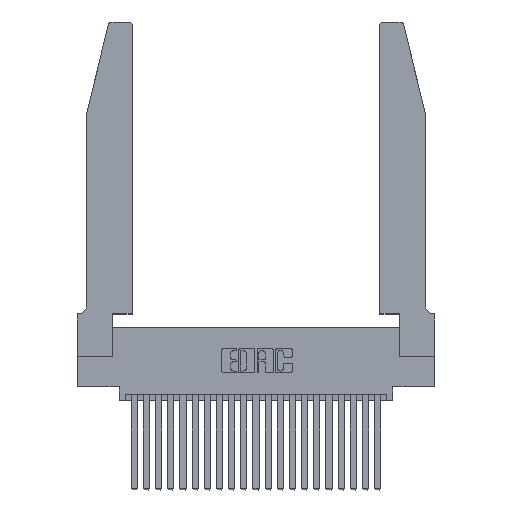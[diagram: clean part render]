
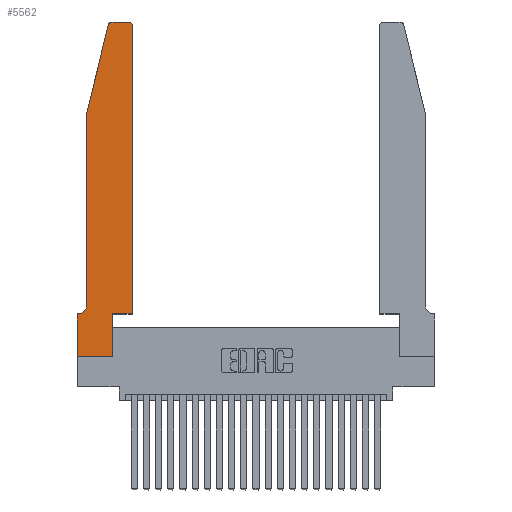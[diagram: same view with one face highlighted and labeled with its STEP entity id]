
A CAD part, top view. The second image highlights one B-rep face of the part: STEP entity #5562.
In plain terms, the highlighted planar face has unit normal (0, 0, 1).
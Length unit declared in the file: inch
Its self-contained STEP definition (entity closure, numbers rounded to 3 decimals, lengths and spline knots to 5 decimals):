
#149 = VECTOR ( 'NONE', #1515, 39.37008 ) ;
#479 = DIRECTION ( 'NONE',  ( 0., 0., 1. ) ) ;
#844 = EDGE_CURVE ( 'NONE', #2425, #8288, #3232, .T. ) ;
#851 = ORIENTED_EDGE ( 'NONE', *, *, #21443, .T. ) ;
#1072 = AXIS2_PLACEMENT_3D ( 'NONE', #11832, #479, #13638 ) ;
#1257 = EDGE_CURVE ( 'NONE', #16092, #20178, #22790, .T. ) ;
#1515 = DIRECTION ( 'NONE',  ( 0., 1., 0. ) ) ;
#1589 = EDGE_CURVE ( 'NONE', #8951, #5964, #16512, .T. ) ;
#1656 = VECTOR ( 'NONE', #19403, 39.37008 ) ;
#2425 = VERTEX_POINT ( 'NONE', #13610 ) ;
#2633 = CARTESIAN_POINT ( 'NONE',  ( 0.4205, 2.72, 0.37 ) ) ;
#2697 = ORIENTED_EDGE ( 'NONE', *, *, #7493, .T. ) ;
#2860 = DIRECTION ( 'NONE',  ( 0., 0., 1. ) ) ;
#3204 = AXIS2_PLACEMENT_3D ( 'NONE', #14001, #2860, #15829 ) ;
#3224 = CIRCLE ( 'NONE', #19484, 0.03 ) ;
#3232 = LINE ( 'NONE', #6905, #16251 ) ;
#3492 = CARTESIAN_POINT ( 'NONE',  ( 0.4505, 0.35, 0.37 ) ) ;
#3588 = VERTEX_POINT ( 'NONE', #11520 ) ;
#3846 = CARTESIAN_POINT ( 'NONE',  ( 0.4505, 0.35, 0.37 ) ) ;
#4590 = DIRECTION ( 'NONE',  ( 1., 0., 0. ) ) ;
#4753 = DIRECTION ( 'NONE',  ( 0., 0., -1. ) ) ;
#5341 = CARTESIAN_POINT ( 'NONE',  ( 0.4205, 2.75, 0.37 ) ) ;
#5562 = ADVANCED_FACE ( 'NONE', ( #9173 ), #22714, .T. ) ;
#5710 = ORIENTED_EDGE ( 'NONE', *, *, #23369, .T. ) ;
#5837 = CARTESIAN_POINT ( 'NONE',  ( 0., 0., 0.37 ) ) ;
#5964 = VERTEX_POINT ( 'NONE', #8178 ) ;
#6214 = CARTESIAN_POINT ( 'NONE',  ( 0.0755, 0.42, 0.37 ) ) ;
#6247 = LINE ( 'NONE', #11692, #10048 ) ;
#6282 = CARTESIAN_POINT ( 'NONE',  ( 0.25487, 2.72718, 0.37 ) ) ;
#6511 = LINE ( 'NONE', #3492, #149 ) ;
#6785 = DIRECTION ( 'NONE',  ( 0., 1., 0. ) ) ;
#6905 = CARTESIAN_POINT ( 'NONE',  ( 0.2865, 0.35, 0.37 ) ) ;
#7107 = LINE ( 'NONE', #5837, #20007 ) ;
#7309 = VERTEX_POINT ( 'NONE', #7958 ) ;
#7493 = EDGE_CURVE ( 'NONE', #22940, #8951, #9661, .T. ) ;
#7734 = ORIENTED_EDGE ( 'NONE', *, *, #1589, .T. ) ;
#7958 = CARTESIAN_POINT ( 'NONE',  ( 0.4505, 0.35, 0.37 ) ) ;
#8178 = CARTESIAN_POINT ( 'NONE',  ( 0., 0.35, 0.37 ) ) ;
#8213 = VECTOR ( 'NONE', #13014, 39.37008 ) ;
#8288 = VERTEX_POINT ( 'NONE', #16744 ) ;
#8327 = ORIENTED_EDGE ( 'NONE', *, *, #11791, .T. ) ;
#8951 = VERTEX_POINT ( 'NONE', #17573 ) ;
#9047 = CARTESIAN_POINT ( 'NONE',  ( 0.0755, 2., 0.37 ) ) ;
#9173 = FACE_OUTER_BOUND ( 'NONE', #22341, .T. ) ;
#9229 = CARTESIAN_POINT ( 'NONE',  ( 0.0755, 2., 0.37 ) ) ;
#9490 = DIRECTION ( 'NONE',  ( 1., 0., 0. ) ) ;
#9661 = CIRCLE ( 'NONE', #21157, 0.07 ) ;
#9697 = CARTESIAN_POINT ( 'NONE',  ( 0.4505, 2.72, 0.37 ) ) ;
#9787 = ORIENTED_EDGE ( 'NONE', *, *, #22344, .T. ) ;
#9845 = DIRECTION ( 'NONE',  ( -1., 0., 0. ) ) ;
#10048 = VECTOR ( 'NONE', #9845, 39.37008 ) ;
#10526 = VECTOR ( 'NONE', #9490, 39.37008 ) ;
#10929 = CIRCLE ( 'NONE', #3204, 0.03 ) ;
#11520 = CARTESIAN_POINT ( 'NONE',  ( 0., 0., 0.37 ) ) ;
#11530 = ORIENTED_EDGE ( 'NONE', *, *, #1257, .T. ) ;
#11692 = CARTESIAN_POINT ( 'NONE',  ( 0.2605, 2.75, 0.37 ) ) ;
#11791 = EDGE_CURVE ( 'NONE', #3588, #2425, #7107, .T. ) ;
#11832 = CARTESIAN_POINT ( 'NONE',  ( 0., 0.35, 0.37 ) ) ;
#12119 = CARTESIAN_POINT ( 'NONE',  ( 0., 0., 0.37 ) ) ;
#12266 = EDGE_CURVE ( 'NONE', #7309, #21883, #6511, .T. ) ;
#12293 = CARTESIAN_POINT ( 'NONE',  ( 0.0755, 0.35, 0.37 ) ) ;
#12650 = ORIENTED_EDGE ( 'NONE', *, *, #12677, .T. ) ;
#12677 = EDGE_CURVE ( 'NONE', #5964, #3588, #14332, .T. ) ;
#12717 = VECTOR ( 'NONE', #22079, 39.37008 ) ;
#13014 = DIRECTION ( 'NONE',  ( -0.239, -0.971, 0. ) ) ;
#13116 = CARTESIAN_POINT ( 'NONE',  ( 0.0755, 2., 0.37 ) ) ;
#13610 = CARTESIAN_POINT ( 'NONE',  ( 0.2865, 0., 0.37 ) ) ;
#13638 = DIRECTION ( 'NONE',  ( 1., 0., 0. ) ) ;
#13783 = ORIENTED_EDGE ( 'NONE', *, *, #15262, .T. ) ;
#14001 = CARTESIAN_POINT ( 'NONE',  ( 0.284, 2.72, 0.37 ) ) ;
#14332 = LINE ( 'NONE', #12119, #23444 ) ;
#14662 = VERTEX_POINT ( 'NONE', #5341 ) ;
#15063 = DIRECTION ( 'NONE',  ( 1., 0., 0. ) ) ;
#15262 = EDGE_CURVE ( 'NONE', #8288, #7309, #20214, .T. ) ;
#15610 = DIRECTION ( 'NONE',  ( 0., 0., 1. ) ) ;
#15739 = DIRECTION ( 'NONE',  ( 0., -1., 0. ) ) ;
#15789 = CARTESIAN_POINT ( 'NONE',  ( 0.0055, 0.42, 0.37 ) ) ;
#15829 = DIRECTION ( 'NONE',  ( 1., 0., 0. ) ) ;
#16092 = VERTEX_POINT ( 'NONE', #6282 ) ;
#16251 = VECTOR ( 'NONE', #6785, 39.37008 ) ;
#16335 = ORIENTED_EDGE ( 'NONE', *, *, #19430, .T. ) ;
#16512 = LINE ( 'NONE', #12293, #1656 ) ;
#16744 = CARTESIAN_POINT ( 'NONE',  ( 0.2865, 0.35, 0.37 ) ) ;
#17573 = CARTESIAN_POINT ( 'NONE',  ( 0.0055, 0.35, 0.37 ) ) ;
#17677 = DIRECTION ( 'NONE',  ( -1., 0., 0. ) ) ;
#18175 = LINE ( 'NONE', #9229, #12717 ) ;
#19231 = ORIENTED_EDGE ( 'NONE', *, *, #12266, .T. ) ;
#19368 = VERTEX_POINT ( 'NONE', #20099 ) ;
#19403 = DIRECTION ( 'NONE',  ( -1., 0., 0. ) ) ;
#19430 = EDGE_CURVE ( 'NONE', #20178, #22940, #18175, .T. ) ;
#19484 = AXIS2_PLACEMENT_3D ( 'NONE', #2633, #15610, #4590 ) ;
#20007 = VECTOR ( 'NONE', #15063, 39.37008 ) ;
#20099 = CARTESIAN_POINT ( 'NONE',  ( 0.284, 2.75, 0.37 ) ) ;
#20178 = VERTEX_POINT ( 'NONE', #13116 ) ;
#20214 = LINE ( 'NONE', #3846, #10526 ) ;
#21157 = AXIS2_PLACEMENT_3D ( 'NONE', #15789, #4753, #17677 ) ;
#21443 = EDGE_CURVE ( 'NONE', #19368, #16092, #10929, .T. ) ;
#21883 = VERTEX_POINT ( 'NONE', #9697 ) ;
#22079 = DIRECTION ( 'NONE',  ( 0., -1., 0. ) ) ;
#22341 = EDGE_LOOP ( 'NONE', ( #9787, #851, #11530, #16335, #2697, #7734, #12650, #8327, #22898, #13783, #19231, #5710 ) ) ;
#22344 = EDGE_CURVE ( 'NONE', #14662, #19368, #6247, .T. ) ;
#22714 = PLANE ( 'NONE',  #1072 ) ;
#22790 = LINE ( 'NONE', #9047, #8213 ) ;
#22898 = ORIENTED_EDGE ( 'NONE', *, *, #844, .T. ) ;
#22940 = VERTEX_POINT ( 'NONE', #6214 ) ;
#23369 = EDGE_CURVE ( 'NONE', #21883, #14662, #3224, .T. ) ;
#23444 = VECTOR ( 'NONE', #15739, 39.37008 ) ;
